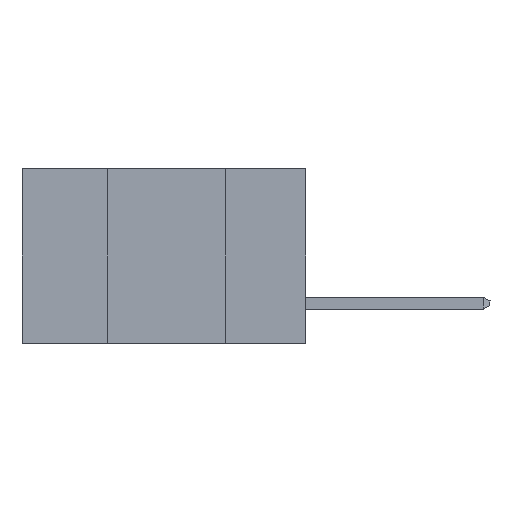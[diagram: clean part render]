
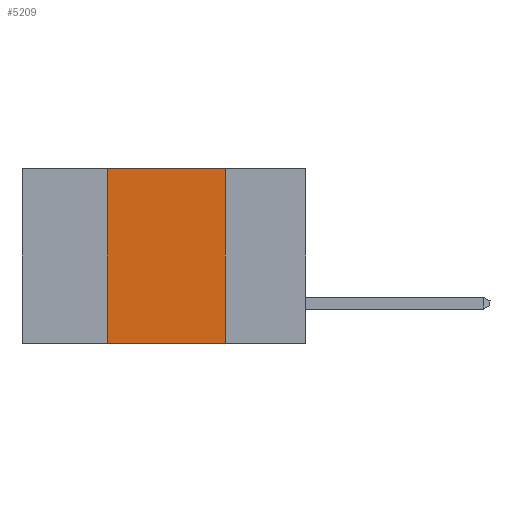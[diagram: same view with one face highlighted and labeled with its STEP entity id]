
A CAD part, left-side view. The second image highlights one B-rep face of the part: STEP entity #5209.
In plain terms, the highlighted planar face has unit normal (-1, 0, 0).
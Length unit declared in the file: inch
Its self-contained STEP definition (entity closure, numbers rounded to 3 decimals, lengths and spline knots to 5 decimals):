
#79 = CARTESIAN_POINT ( 'NONE',  ( 0., 0.6, -0.37 ) ) ;
#1104 = ORIENTED_EDGE ( 'NONE', *, *, #14839, .F. ) ;
#1375 = EDGE_LOOP ( 'NONE', ( #29971, #1104, #6202, #21995 ) ) ;
#2125 = CARTESIAN_POINT ( 'NONE',  ( 0., 0.17, 0. ) ) ;
#3103 = VECTOR ( 'NONE', #10180, 39.37008 ) ;
#3950 = EDGE_CURVE ( 'NONE', #27246, #18620, #29156, .T. ) ;
#4688 = VERTEX_POINT ( 'NONE', #26135 ) ;
#5209 = ADVANCED_FACE ( 'NONE', ( #25830 ), #29359, .F. ) ;
#5800 = VECTOR ( 'NONE', #14144, 39.37008 ) ;
#6202 = ORIENTED_EDGE ( 'NONE', *, *, #21572, .F. ) ;
#7917 = VECTOR ( 'NONE', #18738, 39.37008 ) ;
#10180 = DIRECTION ( 'NONE',  ( 0., -1., 0. ) ) ;
#11175 = CARTESIAN_POINT ( 'NONE',  ( 0., 0.6, 0. ) ) ;
#12791 = CARTESIAN_POINT ( 'NONE',  ( 0., 0.17, 0. ) ) ;
#14144 = DIRECTION ( 'NONE',  ( 0., -1., 0. ) ) ;
#14839 = EDGE_CURVE ( 'NONE', #4688, #29716, #15002, .T. ) ;
#15002 = LINE ( 'NONE', #11175, #5800 ) ;
#16584 = CARTESIAN_POINT ( 'NONE',  ( 0., 0.6, 0. ) ) ;
#16597 = CARTESIAN_POINT ( 'NONE',  ( 0., 0.42, 0. ) ) ;
#18276 = LINE ( 'NONE', #2125, #19101 ) ;
#18620 = VERTEX_POINT ( 'NONE', #22638 ) ;
#18738 = DIRECTION ( 'NONE',  ( 0., 0., 1. ) ) ;
#18834 = DIRECTION ( 'NONE',  ( 0., 0., -1. ) ) ;
#19101 = VECTOR ( 'NONE', #24617, 39.37008 ) ;
#20358 = LINE ( 'NONE', #16597, #7917 ) ;
#21572 = EDGE_CURVE ( 'NONE', #27246, #4688, #20358, .T. ) ;
#21995 = ORIENTED_EDGE ( 'NONE', *, *, #3950, .T. ) ;
#22638 = CARTESIAN_POINT ( 'NONE',  ( 0., 0.17, -0.37 ) ) ;
#23400 = AXIS2_PLACEMENT_3D ( 'NONE', #16584, #29136, #18834 ) ;
#24617 = DIRECTION ( 'NONE',  ( 0., 0., -1. ) ) ;
#25830 = FACE_OUTER_BOUND ( 'NONE', #1375, .T. ) ;
#26135 = CARTESIAN_POINT ( 'NONE',  ( 0., 0.42, 0. ) ) ;
#27246 = VERTEX_POINT ( 'NONE', #33169 ) ;
#29136 = DIRECTION ( 'NONE',  ( 1., 0., 0. ) ) ;
#29156 = LINE ( 'NONE', #79, #3103 ) ;
#29277 = EDGE_CURVE ( 'NONE', #29716, #18620, #18276, .T. ) ;
#29359 = PLANE ( 'NONE',  #23400 ) ;
#29716 = VERTEX_POINT ( 'NONE', #12791 ) ;
#29971 = ORIENTED_EDGE ( 'NONE', *, *, #29277, .F. ) ;
#33169 = CARTESIAN_POINT ( 'NONE',  ( 0., 0.42, -0.37 ) ) ;
